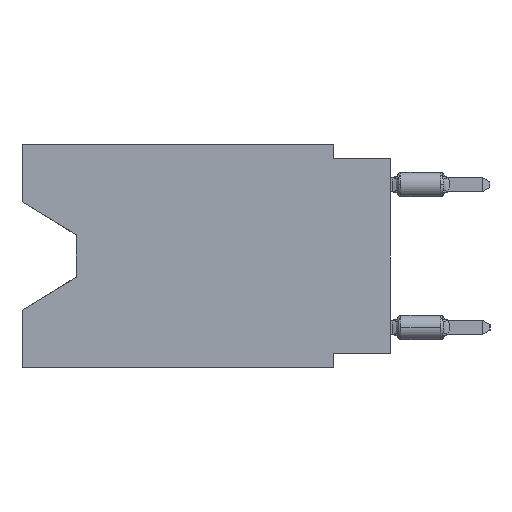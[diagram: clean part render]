
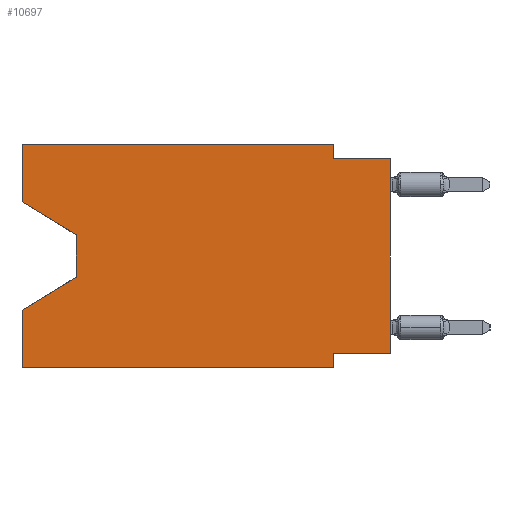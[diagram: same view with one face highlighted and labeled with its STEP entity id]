
A CAD part, left-side view. The second image highlights one B-rep face of the part: STEP entity #10697.
In plain terms, the highlighted planar face has unit normal (-1, 0, 0).
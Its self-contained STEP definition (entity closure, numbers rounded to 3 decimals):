
#74 = VECTOR ( 'NONE', #29144, 1000. ) ;
#1400 = EDGE_CURVE ( 'NONE', #7922, #16577, #6444, .T. ) ;
#1742 = VECTOR ( 'NONE', #8816, 1000. ) ;
#3333 = CARTESIAN_POINT ( 'NONE',  ( 0., 2.54, -9.906 ) ) ;
#3447 = CARTESIAN_POINT ( 'NONE',  ( 0., 16.383, 0. ) ) ;
#5341 = CARTESIAN_POINT ( 'NONE',  ( 0., 13.97, -4.013 ) ) ;
#5472 = ORIENTED_EDGE ( 'NONE', *, *, #18458, .F. ) ;
#5808 = LINE ( 'NONE', #39862, #14435 ) ;
#6190 = ORIENTED_EDGE ( 'NONE', *, *, #8544, .T. ) ;
#6444 = LINE ( 'NONE', #33617, #43426 ) ;
#7922 = VERTEX_POINT ( 'NONE', #34401 ) ;
#8165 = LINE ( 'NONE', #19041, #1742 ) ;
#8390 = CARTESIAN_POINT ( 'NONE',  ( 0., 16.383, 0. ) ) ;
#8544 = EDGE_CURVE ( 'NONE', #23613, #10087, #5808, .T. ) ;
#8591 = DIRECTION ( 'NONE',  ( 0., 0., 1. ) ) ;
#8747 = VERTEX_POINT ( 'NONE', #3333 ) ;
#8816 = DIRECTION ( 'NONE',  ( 0., 0., 1. ) ) ;
#9308 = CARTESIAN_POINT ( 'NONE',  ( 0., 0., -9.271 ) ) ;
#9431 = CARTESIAN_POINT ( 'NONE',  ( 0., 2.54, -9.271 ) ) ;
#9625 = CARTESIAN_POINT ( 'NONE',  ( 0., 16.383, -9.906 ) ) ;
#10054 = VECTOR ( 'NONE', #21209, 1000. ) ;
#10087 = VERTEX_POINT ( 'NONE', #41199 ) ;
#10206 = VERTEX_POINT ( 'NONE', #9308 ) ;
#10256 = VERTEX_POINT ( 'NONE', #32925 ) ;
#10697 = ADVANCED_FACE ( 'NONE', ( #32872 ), #11949, .F. ) ;
#11160 = VERTEX_POINT ( 'NONE', #16051 ) ;
#11266 = VECTOR ( 'NONE', #29951, 1000. ) ;
#11407 = LINE ( 'NONE', #32110, #10054 ) ;
#11683 = LINE ( 'NONE', #21046, #19074 ) ;
#11833 = CARTESIAN_POINT ( 'NONE',  ( 0., 2.54, -0.635 ) ) ;
#11949 = PLANE ( 'NONE',  #25843 ) ;
#11958 = ORIENTED_EDGE ( 'NONE', *, *, #13281, .T. ) ;
#12690 = CARTESIAN_POINT ( 'NONE',  ( 0., 2.54, 0. ) ) ;
#12755 = EDGE_CURVE ( 'NONE', #22122, #8747, #11407, .T. ) ;
#13281 = EDGE_CURVE ( 'NONE', #10087, #7922, #22249, .T. ) ;
#13590 = VECTOR ( 'NONE', #41428, 1000. ) ;
#14024 = LINE ( 'NONE', #27612, #13590 ) ;
#14435 = VECTOR ( 'NONE', #32101, 1000. ) ;
#15088 = DIRECTION ( 'NONE',  ( 0., 0., -1. ) ) ;
#15769 = VECTOR ( 'NONE', #8591, 1000. ) ;
#16051 = CARTESIAN_POINT ( 'NONE',  ( 0., 0., -0.635 ) ) ;
#16577 = VERTEX_POINT ( 'NONE', #28345 ) ;
#16758 = CARTESIAN_POINT ( 'NONE',  ( 0., 16.383, 0. ) ) ;
#16907 = LINE ( 'NONE', #12690, #37252 ) ;
#17024 = DIRECTION ( 'NONE',  ( 0., 0., 1. ) ) ;
#18137 = DIRECTION ( 'NONE',  ( 0., 1., 0. ) ) ;
#18168 = LINE ( 'NONE', #32400, #15769 ) ;
#18334 = VERTEX_POINT ( 'NONE', #11833 ) ;
#18354 = DIRECTION ( 'NONE',  ( 0., -1., 0. ) ) ;
#18458 = EDGE_CURVE ( 'NONE', #10256, #18334, #16907, .T. ) ;
#19041 = CARTESIAN_POINT ( 'NONE',  ( 0., 0., 0. ) ) ;
#19074 = VECTOR ( 'NONE', #18354, 1000. ) ;
#19118 = EDGE_CURVE ( 'NONE', #10206, #11160, #8165, .T. ) ;
#19516 = ORIENTED_EDGE ( 'NONE', *, *, #41163, .F. ) ;
#19651 = ORIENTED_EDGE ( 'NONE', *, *, #42054, .F. ) ;
#21046 = CARTESIAN_POINT ( 'NONE',  ( 0., 0., -0.635 ) ) ;
#21209 = DIRECTION ( 'NONE',  ( 0., -1., 0. ) ) ;
#21486 = CARTESIAN_POINT ( 'NONE',  ( 0., 0., -9.271 ) ) ;
#21501 = ORIENTED_EDGE ( 'NONE', *, *, #19118, .T. ) ;
#21570 = EDGE_CURVE ( 'NONE', #23613, #31498, #18168, .T. ) ;
#22122 = VERTEX_POINT ( 'NONE', #9625 ) ;
#22249 = LINE ( 'NONE', #5341, #74 ) ;
#23138 = EDGE_CURVE ( 'NONE', #22122, #16577, #31491, .T. ) ;
#23613 = VERTEX_POINT ( 'NONE', #34074 ) ;
#24835 = VERTEX_POINT ( 'NONE', #9431 ) ;
#25843 = AXIS2_PLACEMENT_3D ( 'NONE', #8390, #29522, #15088 ) ;
#26726 = ORIENTED_EDGE ( 'NONE', *, *, #35927, .F. ) ;
#27222 = VECTOR ( 'NONE', #17024, 1000. ) ;
#27610 = VECTOR ( 'NONE', #18137, 1000. ) ;
#27612 = CARTESIAN_POINT ( 'NONE',  ( 0., 2.54, -9.906 ) ) ;
#28154 = LINE ( 'NONE', #21486, #27610 ) ;
#28345 = CARTESIAN_POINT ( 'NONE',  ( 0., 16.383, -7.36 ) ) ;
#29144 = DIRECTION ( 'NONE',  ( 0., 0., -1. ) ) ;
#29522 = DIRECTION ( 'NONE',  ( 1., 0., 0. ) ) ;
#29951 = DIRECTION ( 'NONE',  ( 0., -1., 0. ) ) ;
#30214 = EDGE_LOOP ( 'NONE', ( #6190, #11958, #38434, #30634, #34892, #19516, #26726, #21501, #19651, #5472, #35072, #32029 ) ) ;
#30634 = ORIENTED_EDGE ( 'NONE', *, *, #23138, .F. ) ;
#31491 = LINE ( 'NONE', #3447, #27222 ) ;
#31498 = VERTEX_POINT ( 'NONE', #16758 ) ;
#32029 = ORIENTED_EDGE ( 'NONE', *, *, #21570, .F. ) ;
#32101 = DIRECTION ( 'NONE',  ( 0., -0.855, -0.519 ) ) ;
#32110 = CARTESIAN_POINT ( 'NONE',  ( 0., 16.383, -9.906 ) ) ;
#32400 = CARTESIAN_POINT ( 'NONE',  ( 0., 16.383, 0. ) ) ;
#32872 = FACE_OUTER_BOUND ( 'NONE', #30214, .T. ) ;
#32925 = CARTESIAN_POINT ( 'NONE',  ( 0., 2.54, 0. ) ) ;
#33389 = DIRECTION ( 'NONE',  ( 0., 0., -1. ) ) ;
#33617 = CARTESIAN_POINT ( 'NONE',  ( 0., 13.97, -5.893 ) ) ;
#34074 = CARTESIAN_POINT ( 'NONE',  ( 0., 16.383, -2.546 ) ) ;
#34401 = CARTESIAN_POINT ( 'NONE',  ( 0., 13.97, -5.893 ) ) ;
#34414 = LINE ( 'NONE', #40871, #11266 ) ;
#34892 = ORIENTED_EDGE ( 'NONE', *, *, #12755, .T. ) ;
#35072 = ORIENTED_EDGE ( 'NONE', *, *, #41989, .F. ) ;
#35927 = EDGE_CURVE ( 'NONE', #10206, #24835, #28154, .T. ) ;
#37252 = VECTOR ( 'NONE', #33389, 1000. ) ;
#38434 = ORIENTED_EDGE ( 'NONE', *, *, #1400, .T. ) ;
#39862 = CARTESIAN_POINT ( 'NONE',  ( 0., 16.383, -2.546 ) ) ;
#40871 = CARTESIAN_POINT ( 'NONE',  ( 0., 16.383, 0. ) ) ;
#41163 = EDGE_CURVE ( 'NONE', #24835, #8747, #14024, .T. ) ;
#41199 = CARTESIAN_POINT ( 'NONE',  ( 0., 13.97, -4.013 ) ) ;
#41428 = DIRECTION ( 'NONE',  ( 0., 0., -1. ) ) ;
#41989 = EDGE_CURVE ( 'NONE', #31498, #10256, #34414, .T. ) ;
#42054 = EDGE_CURVE ( 'NONE', #18334, #11160, #11683, .T. ) ;
#43401 = DIRECTION ( 'NONE',  ( 0., 0.855, -0.519 ) ) ;
#43426 = VECTOR ( 'NONE', #43401, 1000. ) ;
